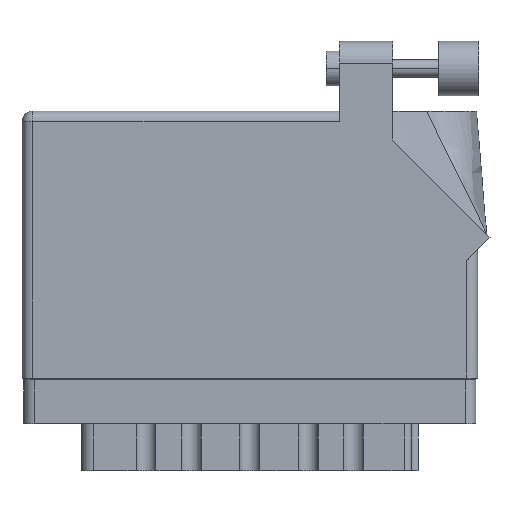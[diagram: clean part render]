
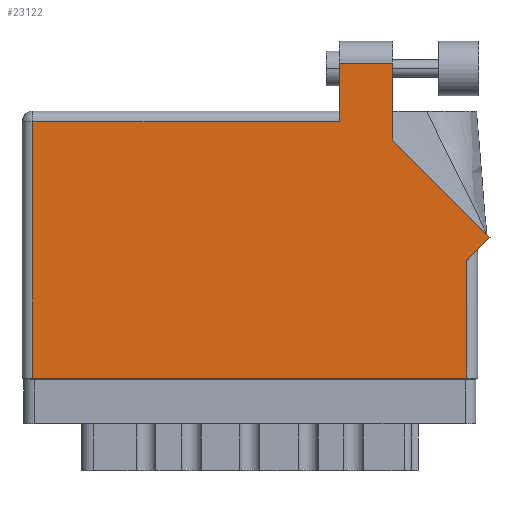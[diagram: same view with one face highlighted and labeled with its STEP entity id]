
A CAD part, front view. The second image highlights one B-rep face of the part: STEP entity #23122.
In plain terms, the highlighted face is planar.
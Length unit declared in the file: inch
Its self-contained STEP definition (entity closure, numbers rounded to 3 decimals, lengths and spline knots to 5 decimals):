
#961 = ORIENTED_EDGE ( 'NONE', *, *, #26390, .T. ) ;
#1512 = LINE ( 'NONE', #33124, #41562 ) ;
#2346 = ORIENTED_EDGE ( 'NONE', *, *, #7704, .T. ) ;
#2533 = VERTEX_POINT ( 'NONE', #6608 ) ;
#2785 = VECTOR ( 'NONE', #39333, 39.37008 ) ;
#2916 = CARTESIAN_POINT ( 'NONE',  ( 0., 1.468, 0. ) ) ;
#4304 = DIRECTION ( 'NONE',  ( 0., -1., 0. ) ) ;
#5138 = LINE ( 'NONE', #41778, #27275 ) ;
#5660 = CARTESIAN_POINT ( 'NONE',  ( 0.062, 0., 0. ) ) ;
#6608 = CARTESIAN_POINT ( 'NONE',  ( 1.819, 1.805, 0. ) ) ;
#6714 = DIRECTION ( 'NONE',  ( 1., 0., 0. ) ) ;
#7272 = CARTESIAN_POINT ( 'NONE',  ( 2.68271, 0.80771, 0. ) ) ;
#7647 = EDGE_CURVE ( 'NONE', #21549, #26097, #42754, .T. ) ;
#7704 = EDGE_CURVE ( 'NONE', #11172, #2533, #12965, .T. ) ;
#8475 = CARTESIAN_POINT ( 'NONE',  ( 0.062, 0., 0. ) ) ;
#8548 = PLANE ( 'NONE',  #34811 ) ;
#8639 = CARTESIAN_POINT ( 'NONE',  ( 1.819, 1.805, 0. ) ) ;
#8706 = DIRECTION ( 'NONE',  ( 0., 0., -1. ) ) ;
#9143 = ORIENTED_EDGE ( 'NONE', *, *, #15020, .T. ) ;
#10228 = VERTEX_POINT ( 'NONE', #38400 ) ;
#10889 = EDGE_LOOP ( 'NONE', ( #48978, #2346, #961, #45274, #40623, #26031, #27450, #11869, #9143 ) ) ;
#11025 = DIRECTION ( 'NONE',  ( 0., 1., 0. ) ) ;
#11172 = VERTEX_POINT ( 'NONE', #44815 ) ;
#11869 = ORIENTED_EDGE ( 'NONE', *, *, #15095, .T. ) ;
#12965 = LINE ( 'NONE', #8639, #2785 ) ;
#13802 = DIRECTION ( 'NONE',  ( -1., 0., 0. ) ) ;
#14479 = CARTESIAN_POINT ( 'NONE',  ( 0.062, 1.468, 0. ) ) ;
#15020 = EDGE_CURVE ( 'NONE', #45927, #41315, #1512, .T. ) ;
#15095 = EDGE_CURVE ( 'NONE', #36297, #45927, #5138, .T. ) ;
#15472 = VECTOR ( 'NONE', #32882, 39.37008 ) ;
#18225 = CARTESIAN_POINT ( 'NONE',  ( 0., 0., 0. ) ) ;
#19613 = LINE ( 'NONE', #2916, #30986 ) ;
#20232 = CARTESIAN_POINT ( 'NONE',  ( 0., 1.53, 0. ) ) ;
#20595 = LINE ( 'NONE', #26575, #37943 ) ;
#21549 = VERTEX_POINT ( 'NONE', #14479 ) ;
#23062 = CARTESIAN_POINT ( 'NONE',  ( 2.126, 1.36442, 0. ) ) ;
#23122 = ADVANCED_FACE ( 'NONE', ( #45965 ), #8548, .F. ) ;
#24201 = DIRECTION ( 'NONE',  ( 0., -1., 0. ) ) ;
#26031 = ORIENTED_EDGE ( 'NONE', *, *, #31962, .T. ) ;
#26097 = VERTEX_POINT ( 'NONE', #5660 ) ;
#26390 = EDGE_CURVE ( 'NONE', #2533, #10228, #20595, .T. ) ;
#26575 = CARTESIAN_POINT ( 'NONE',  ( 1.819, 1.53, 0. ) ) ;
#26655 = DIRECTION ( 'NONE',  ( 0.707, 0.707, 0. ) ) ;
#26877 = LINE ( 'NONE', #28431, #15472 ) ;
#27275 = VECTOR ( 'NONE', #26655, 39.37008 ) ;
#27450 = ORIENTED_EDGE ( 'NONE', *, *, #34065, .T. ) ;
#28431 = CARTESIAN_POINT ( 'NONE',  ( 2.55, 0.737, 0. ) ) ;
#28773 = VECTOR ( 'NONE', #6714, 39.37008 ) ;
#29947 = EDGE_CURVE ( 'NONE', #41315, #11172, #42398, .T. ) ;
#30986 = VECTOR ( 'NONE', #13802, 39.37008 ) ;
#31701 = CARTESIAN_POINT ( 'NONE',  ( 2.126, 1.36442, 0. ) ) ;
#31962 = EDGE_CURVE ( 'NONE', #26097, #41692, #38894, .T. ) ;
#32882 = DIRECTION ( 'NONE',  ( 0., 1., 0. ) ) ;
#33124 = CARTESIAN_POINT ( 'NONE',  ( 2.68271, 0.80771, 0. ) ) ;
#33794 = DIRECTION ( 'NONE',  ( -0.707, 0.707, 0. ) ) ;
#34065 = EDGE_CURVE ( 'NONE', #41692, #36297, #26877, .T. ) ;
#34811 = AXIS2_PLACEMENT_3D ( 'NONE', #20232, #8706, #42585 ) ;
#36140 = CARTESIAN_POINT ( 'NONE',  ( 2.55, 0.675, 0. ) ) ;
#36297 = VERTEX_POINT ( 'NONE', #36140 ) ;
#37410 = VECTOR ( 'NONE', #24201, 39.37008 ) ;
#37943 = VECTOR ( 'NONE', #4304, 39.37008 ) ;
#38400 = CARTESIAN_POINT ( 'NONE',  ( 1.819, 1.468, 0. ) ) ;
#38894 = LINE ( 'NONE', #18225, #28773 ) ;
#39333 = DIRECTION ( 'NONE',  ( -1., 0., 0. ) ) ;
#39804 = EDGE_CURVE ( 'NONE', #10228, #21549, #19613, .T. ) ;
#40623 = ORIENTED_EDGE ( 'NONE', *, *, #7647, .T. ) ;
#41315 = VERTEX_POINT ( 'NONE', #31701 ) ;
#41562 = VECTOR ( 'NONE', #33794, 39.37008 ) ;
#41692 = VERTEX_POINT ( 'NONE', #49005 ) ;
#41778 = CARTESIAN_POINT ( 'NONE',  ( 2.612, 0.737, 0. ) ) ;
#42398 = LINE ( 'NONE', #23062, #49533 ) ;
#42585 = DIRECTION ( 'NONE',  ( -1., 0., 0. ) ) ;
#42754 = LINE ( 'NONE', #8475, #37410 ) ;
#44815 = CARTESIAN_POINT ( 'NONE',  ( 2.126, 1.805, 0. ) ) ;
#45274 = ORIENTED_EDGE ( 'NONE', *, *, #39804, .T. ) ;
#45927 = VERTEX_POINT ( 'NONE', #7272 ) ;
#45965 = FACE_OUTER_BOUND ( 'NONE', #10889, .T. ) ;
#48978 = ORIENTED_EDGE ( 'NONE', *, *, #29947, .T. ) ;
#49005 = CARTESIAN_POINT ( 'NONE',  ( 2.55, 0., 0. ) ) ;
#49533 = VECTOR ( 'NONE', #11025, 39.37008 ) ;
